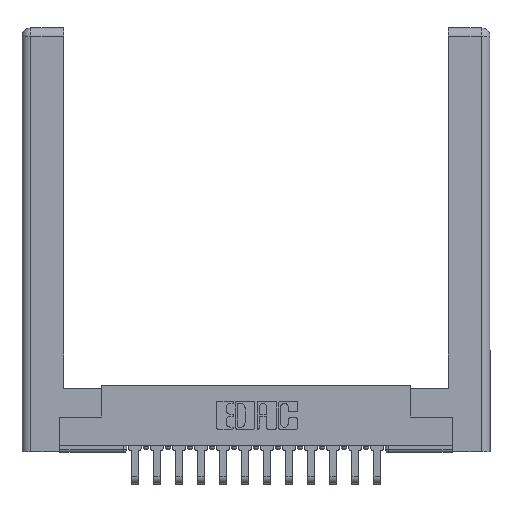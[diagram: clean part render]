
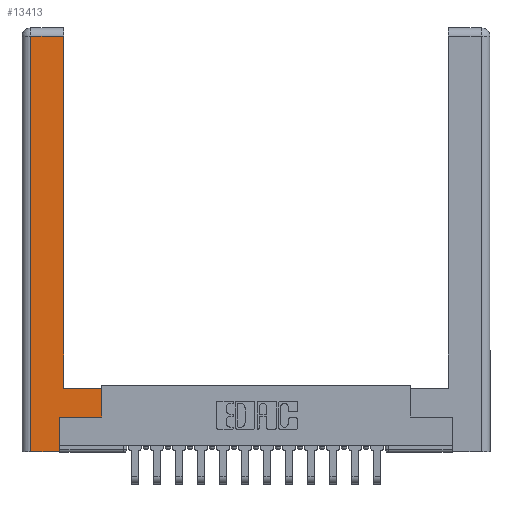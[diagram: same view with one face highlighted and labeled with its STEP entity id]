
A CAD part, top view. The second image highlights one B-rep face of the part: STEP entity #13413.
In plain terms, the highlighted planar face has unit normal (0, 0, 1).
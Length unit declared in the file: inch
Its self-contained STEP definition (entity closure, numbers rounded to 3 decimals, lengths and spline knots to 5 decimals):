
#985 = CARTESIAN_POINT ( 'NONE',  ( 0.565, 0.245, 0. ) ) ;
#1020 = DIRECTION ( 'NONE',  ( 1., 0., 0. ) ) ;
#1247 = VECTOR ( 'NONE', #18137, 39.37008 ) ;
#1263 = LINE ( 'NONE', #5153, #9361 ) ;
#1775 = CARTESIAN_POINT ( 'NONE',  ( 0.295, 3., 0. ) ) ;
#1949 = CARTESIAN_POINT ( 'NONE',  ( 0.265, 0.245, 0. ) ) ;
#2292 = ORIENTED_EDGE ( 'NONE', *, *, #10135, .T. ) ;
#2663 = CARTESIAN_POINT ( 'NONE',  ( 0., 0., 0. ) ) ;
#2722 = VERTEX_POINT ( 'NONE', #10481 ) ;
#2875 = DIRECTION ( 'NONE',  ( 0., -1., 0. ) ) ;
#3802 = VERTEX_POINT ( 'NONE', #985 ) ;
#3859 = ORIENTED_EDGE ( 'NONE', *, *, #16868, .T. ) ;
#4037 = CARTESIAN_POINT ( 'NONE',  ( 0.0615, 2.94, 0. ) ) ;
#4070 = DIRECTION ( 'NONE',  ( 0., 0., -1. ) ) ;
#4651 = LINE ( 'NONE', #14355, #16028 ) ;
#5153 = CARTESIAN_POINT ( 'NONE',  ( 0.295, 0.45, 0. ) ) ;
#5193 = CARTESIAN_POINT ( 'NONE',  ( 0.565, 0.245, 0. ) ) ;
#5436 = LINE ( 'NONE', #9733, #13045 ) ;
#5482 = CARTESIAN_POINT ( 'NONE',  ( 0.295, 0.45, 0. ) ) ;
#6746 = EDGE_CURVE ( 'NONE', #3802, #13309, #15238, .T. ) ;
#6750 = CARTESIAN_POINT ( 'NONE',  ( 0.565, 0.45, 0. ) ) ;
#7435 = ORIENTED_EDGE ( 'NONE', *, *, #18079, .T. ) ;
#7464 = EDGE_LOOP ( 'NONE', ( #12147, #14061, #15319, #2292, #3859, #7435, #8761, #12742 ) ) ;
#7534 = EDGE_CURVE ( 'NONE', #15876, #2722, #12805, .T. ) ;
#8162 = EDGE_CURVE ( 'NONE', #10679, #15876, #14560, .T. ) ;
#8271 = PLANE ( 'NONE',  #11938 ) ;
#8503 = CARTESIAN_POINT ( 'NONE',  ( 0.265, 0., 0. ) ) ;
#8636 = VERTEX_POINT ( 'NONE', #10199 ) ;
#8761 = ORIENTED_EDGE ( 'NONE', *, *, #6746, .T. ) ;
#9114 = CARTESIAN_POINT ( 'NONE',  ( 0.565, 0.45, 0. ) ) ;
#9361 = VECTOR ( 'NONE', #13760, 39.37008 ) ;
#9478 = CARTESIAN_POINT ( 'NONE',  ( 0.295, 2.94, 0. ) ) ;
#9733 = CARTESIAN_POINT ( 'NONE',  ( 0.265, 0., 0. ) ) ;
#9924 = EDGE_CURVE ( 'NONE', #2722, #8636, #4651, .T. ) ;
#10135 = EDGE_CURVE ( 'NONE', #8636, #15710, #5436, .T. ) ;
#10199 = CARTESIAN_POINT ( 'NONE',  ( 0.0615, 0., 0. ) ) ;
#10300 = DIRECTION ( 'NONE',  ( 0., 1., 0. ) ) ;
#10481 = CARTESIAN_POINT ( 'NONE',  ( 0.0615, 2.94, 0. ) ) ;
#10679 = VERTEX_POINT ( 'NONE', #5482 ) ;
#11938 = AXIS2_PLACEMENT_3D ( 'NONE', #2663, #4070, #13967 ) ;
#12147 = ORIENTED_EDGE ( 'NONE', *, *, #8162, .T. ) ;
#12569 = CARTESIAN_POINT ( 'NONE',  ( 0.265, 0.245, 0. ) ) ;
#12638 = VECTOR ( 'NONE', #10300, 39.37008 ) ;
#12742 = ORIENTED_EDGE ( 'NONE', *, *, #17235, .T. ) ;
#12805 = LINE ( 'NONE', #4037, #13191 ) ;
#13045 = VECTOR ( 'NONE', #16952, 39.37008 ) ;
#13161 = DIRECTION ( 'NONE',  ( 0., 1., 0. ) ) ;
#13191 = VECTOR ( 'NONE', #13834, 39.37008 ) ;
#13309 = VERTEX_POINT ( 'NONE', #9114 ) ;
#13413 = ADVANCED_FACE ( 'NONE', ( #15364 ), #8271, .F. ) ;
#13760 = DIRECTION ( 'NONE',  ( -1., 0., 0. ) ) ;
#13834 = DIRECTION ( 'NONE',  ( -1., 0., 0. ) ) ;
#13967 = DIRECTION ( 'NONE',  ( -1., 0., 0. ) ) ;
#14061 = ORIENTED_EDGE ( 'NONE', *, *, #7534, .T. ) ;
#14084 = LINE ( 'NONE', #12569, #12638 ) ;
#14355 = CARTESIAN_POINT ( 'NONE',  ( 0.0615, 0., 0. ) ) ;
#14560 = LINE ( 'NONE', #1775, #15506 ) ;
#14779 = VECTOR ( 'NONE', #1020, 39.37008 ) ;
#15107 = VERTEX_POINT ( 'NONE', #1949 ) ;
#15238 = LINE ( 'NONE', #6750, #1247 ) ;
#15319 = ORIENTED_EDGE ( 'NONE', *, *, #9924, .T. ) ;
#15364 = FACE_OUTER_BOUND ( 'NONE', #7464, .T. ) ;
#15506 = VECTOR ( 'NONE', #13161, 39.37008 ) ;
#15710 = VERTEX_POINT ( 'NONE', #8503 ) ;
#15876 = VERTEX_POINT ( 'NONE', #9478 ) ;
#16028 = VECTOR ( 'NONE', #2875, 39.37008 ) ;
#16868 = EDGE_CURVE ( 'NONE', #15710, #15107, #14084, .T. ) ;
#16952 = DIRECTION ( 'NONE',  ( 1., 0., 0. ) ) ;
#17235 = EDGE_CURVE ( 'NONE', #13309, #10679, #1263, .T. ) ;
#17849 = LINE ( 'NONE', #5193, #14779 ) ;
#18079 = EDGE_CURVE ( 'NONE', #15107, #3802, #17849, .T. ) ;
#18137 = DIRECTION ( 'NONE',  ( 0., 1., 0. ) ) ;
